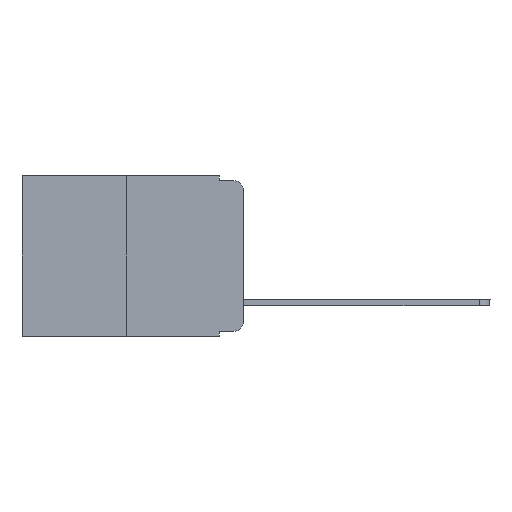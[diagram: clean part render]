
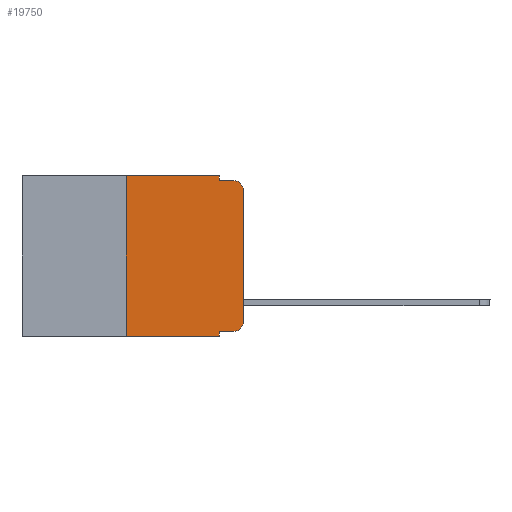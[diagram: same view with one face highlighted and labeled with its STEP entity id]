
A CAD part, left-side view. The second image highlights one B-rep face of the part: STEP entity #19750.
In plain terms, the highlighted planar face has unit normal (-1, 0, 0).
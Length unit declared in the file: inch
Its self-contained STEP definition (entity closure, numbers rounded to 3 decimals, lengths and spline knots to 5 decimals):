
#127 = ORIENTED_EDGE ( 'NONE', *, *, #8685, .F. ) ;
#199 = LINE ( 'NONE', #17397, #9025 ) ;
#711 = AXIS2_PLACEMENT_3D ( 'NONE', #1796, #20257, #15552 ) ;
#863 = CARTESIAN_POINT ( 'NONE',  ( 0., 0., -0.03 ) ) ;
#1136 = VERTEX_POINT ( 'NONE', #863 ) ;
#1673 = EDGE_CURVE ( 'NONE', #9835, #9459, #3552, .T. ) ;
#1796 = CARTESIAN_POINT ( 'NONE',  ( 0., 0.02, -0.03 ) ) ;
#1857 = CIRCLE ( 'NONE', #18233, 0.02 ) ;
#1913 = VERTEX_POINT ( 'NONE', #13065 ) ;
#1975 = CARTESIAN_POINT ( 'NONE',  ( 0., 0.02, -0.313 ) ) ;
#1982 = DIRECTION ( 'NONE',  ( 0., 0., -1. ) ) ;
#2371 = ORIENTED_EDGE ( 'NONE', *, *, #11415, .F. ) ;
#2988 = ORIENTED_EDGE ( 'NONE', *, *, #12642, .F. ) ;
#3175 = DIRECTION ( 'NONE',  ( 0., 0., -1. ) ) ;
#3226 = CARTESIAN_POINT ( 'NONE',  ( 0., 0.051, 0. ) ) ;
#3294 = EDGE_CURVE ( 'NONE', #8307, #17548, #1857, .T. ) ;
#3434 = CARTESIAN_POINT ( 'NONE',  ( 0., 0., -0.313 ) ) ;
#3552 = LINE ( 'NONE', #17596, #13236 ) ;
#3945 = DIRECTION ( 'NONE',  ( 0., 0., 1. ) ) ;
#4063 = DIRECTION ( 'NONE',  ( 0., 0., 1. ) ) ;
#4174 = CARTESIAN_POINT ( 'NONE',  ( 0., 0.051, -0.333 ) ) ;
#4479 = CARTESIAN_POINT ( 'NONE',  ( 0., 0.473, -0.343 ) ) ;
#4613 = CARTESIAN_POINT ( 'NONE',  ( 0., 0.051, 0. ) ) ;
#4667 = EDGE_CURVE ( 'NONE', #10259, #8307, #19641, .T. ) ;
#4731 = EDGE_CURVE ( 'NONE', #6972, #10717, #9462, .T. ) ;
#5603 = LINE ( 'NONE', #18109, #15592 ) ;
#6001 = ORIENTED_EDGE ( 'NONE', *, *, #1673, .F. ) ;
#6972 = VERTEX_POINT ( 'NONE', #9512 ) ;
#7215 = EDGE_CURVE ( 'NONE', #1136, #1913, #12482, .T. ) ;
#8288 = VECTOR ( 'NONE', #3945, 39.37008 ) ;
#8307 = VERTEX_POINT ( 'NONE', #9892 ) ;
#8661 = VERTEX_POINT ( 'NONE', #12543 ) ;
#8685 = EDGE_CURVE ( 'NONE', #10259, #10717, #19208, .T. ) ;
#8938 = VECTOR ( 'NONE', #1982, 39.37008 ) ;
#8990 = PLANE ( 'NONE',  #15863 ) ;
#9025 = VECTOR ( 'NONE', #14020, 39.37008 ) ;
#9459 = VERTEX_POINT ( 'NONE', #16824 ) ;
#9462 = LINE ( 'NONE', #4479, #19665 ) ;
#9512 = CARTESIAN_POINT ( 'NONE',  ( 0., 0.25, -0.343 ) ) ;
#9835 = VERTEX_POINT ( 'NONE', #13282 ) ;
#9892 = CARTESIAN_POINT ( 'NONE',  ( 0., 0.02, -0.333 ) ) ;
#10259 = VERTEX_POINT ( 'NONE', #19409 ) ;
#10479 = CARTESIAN_POINT ( 'NONE',  ( 0., 0.25, 0. ) ) ;
#10717 = VERTEX_POINT ( 'NONE', #18267 ) ;
#11415 = EDGE_CURVE ( 'NONE', #8661, #1913, #199, .T. ) ;
#11626 = VECTOR ( 'NONE', #3175, 39.37008 ) ;
#11962 = FACE_OUTER_BOUND ( 'NONE', #13021, .T. ) ;
#12482 = CIRCLE ( 'NONE', #711, 0.02 ) ;
#12543 = CARTESIAN_POINT ( 'NONE',  ( 0., 0.051, -0.01 ) ) ;
#12642 = EDGE_CURVE ( 'NONE', #9459, #8661, #14027, .T. ) ;
#12985 = ORIENTED_EDGE ( 'NONE', *, *, #18940, .F. ) ;
#13021 = EDGE_LOOP ( 'NONE', ( #16005, #20094, #2371, #2988, #6001, #12985, #19172, #127, #20224, #13439 ) ) ;
#13065 = CARTESIAN_POINT ( 'NONE',  ( 0., 0.02, -0.01 ) ) ;
#13236 = VECTOR ( 'NONE', #18820, 39.37008 ) ;
#13282 = CARTESIAN_POINT ( 'NONE',  ( 0., 0.25, 0. ) ) ;
#13347 = EDGE_CURVE ( 'NONE', #17548, #1136, #5603, .T. ) ;
#13439 = ORIENTED_EDGE ( 'NONE', *, *, #3294, .T. ) ;
#13480 = DIRECTION ( 'NONE',  ( 0., -1., 0. ) ) ;
#13789 = DIRECTION ( 'NONE',  ( 0., 0., -1. ) ) ;
#14020 = DIRECTION ( 'NONE',  ( 0., -1., 0. ) ) ;
#14027 = LINE ( 'NONE', #4613, #11626 ) ;
#15544 = DIRECTION ( 'NONE',  ( 0., -1., 0. ) ) ;
#15552 = DIRECTION ( 'NONE',  ( 0., 0., -1. ) ) ;
#15592 = VECTOR ( 'NONE', #4063, 39.37008 ) ;
#15863 = AXIS2_PLACEMENT_3D ( 'NONE', #18231, #16889, #13789 ) ;
#16005 = ORIENTED_EDGE ( 'NONE', *, *, #13347, .T. ) ;
#16824 = CARTESIAN_POINT ( 'NONE',  ( 0., 0.051, 0. ) ) ;
#16889 = DIRECTION ( 'NONE',  ( 1., 0., 0. ) ) ;
#17397 = CARTESIAN_POINT ( 'NONE',  ( 0., 0.051, -0.01 ) ) ;
#17548 = VERTEX_POINT ( 'NONE', #3434 ) ;
#17568 = DIRECTION ( 'NONE',  ( 0., 0., -1. ) ) ;
#17596 = CARTESIAN_POINT ( 'NONE',  ( 0., 0.473, 0. ) ) ;
#17701 = VECTOR ( 'NONE', #13480, 39.37008 ) ;
#18109 = CARTESIAN_POINT ( 'NONE',  ( 0., 0., 0. ) ) ;
#18231 = CARTESIAN_POINT ( 'NONE',  ( 0., 0.473, 0. ) ) ;
#18233 = AXIS2_PLACEMENT_3D ( 'NONE', #1975, #18895, #17568 ) ;
#18267 = CARTESIAN_POINT ( 'NONE',  ( 0., 0.051, -0.343 ) ) ;
#18291 = LINE ( 'NONE', #10479, #8288 ) ;
#18820 = DIRECTION ( 'NONE',  ( 0., -1., 0. ) ) ;
#18895 = DIRECTION ( 'NONE',  ( -1., 0., 0. ) ) ;
#18940 = EDGE_CURVE ( 'NONE', #6972, #9835, #18291, .T. ) ;
#19172 = ORIENTED_EDGE ( 'NONE', *, *, #4731, .T. ) ;
#19208 = LINE ( 'NONE', #3226, #8938 ) ;
#19409 = CARTESIAN_POINT ( 'NONE',  ( 0., 0.051, -0.333 ) ) ;
#19641 = LINE ( 'NONE', #4174, #17701 ) ;
#19665 = VECTOR ( 'NONE', #15544, 39.37008 ) ;
#19750 = ADVANCED_FACE ( 'NONE', ( #11962 ), #8990, .F. ) ;
#20094 = ORIENTED_EDGE ( 'NONE', *, *, #7215, .T. ) ;
#20224 = ORIENTED_EDGE ( 'NONE', *, *, #4667, .T. ) ;
#20257 = DIRECTION ( 'NONE',  ( -1., 0., 0. ) ) ;
